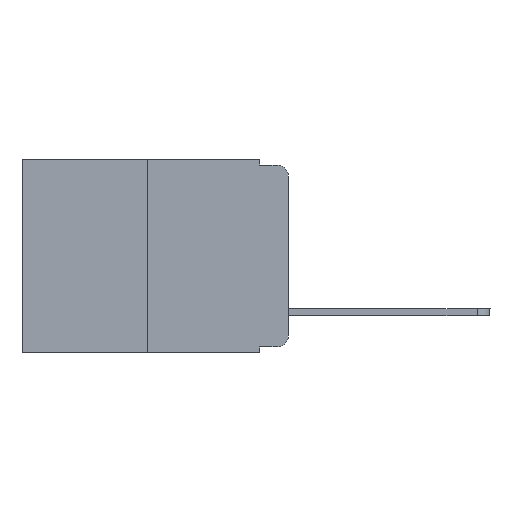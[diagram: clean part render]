
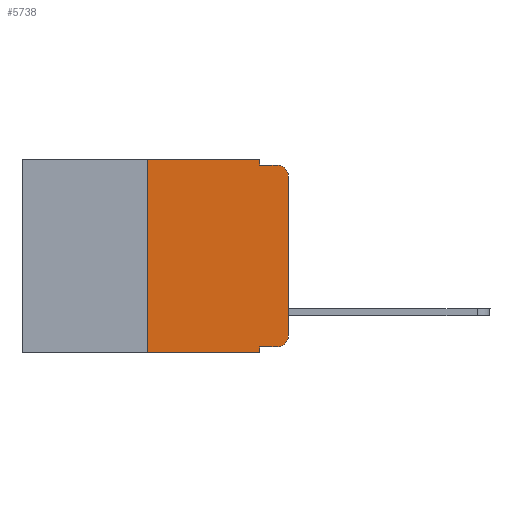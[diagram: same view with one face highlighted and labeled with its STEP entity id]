
A CAD part, left-side view. The second image highlights one B-rep face of the part: STEP entity #5738.
In plain terms, the highlighted planar face has unit normal (-1, 0, 0).
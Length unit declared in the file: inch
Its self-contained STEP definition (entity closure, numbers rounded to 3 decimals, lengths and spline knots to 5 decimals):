
#216 = EDGE_LOOP ( 'NONE', ( #12661, #5060, #540, #6950, #2958, #3601, #13389, #7223, #9988, #9364 ) ) ;
#259 = VECTOR ( 'NONE', #4154, 39.37008 ) ;
#318 = LINE ( 'NONE', #15858, #13446 ) ;
#540 = ORIENTED_EDGE ( 'NONE', *, *, #12259, .F. ) ;
#724 = VECTOR ( 'NONE', #11496, 39.37008 ) ;
#1175 = VERTEX_POINT ( 'NONE', #9957 ) ;
#1369 = VERTEX_POINT ( 'NONE', #2977 ) ;
#1578 = CARTESIAN_POINT ( 'NONE',  ( 0., 0.051, -0.01 ) ) ;
#1842 = EDGE_CURVE ( 'NONE', #11003, #3989, #5611, .T. ) ;
#2008 = LINE ( 'NONE', #15488, #11541 ) ;
#2069 = EDGE_CURVE ( 'NONE', #1369, #3989, #2008, .T. ) ;
#2119 = CARTESIAN_POINT ( 'NONE',  ( 0., 0.473, 0. ) ) ;
#2423 = DIRECTION ( 'NONE',  ( 0., -1., 0. ) ) ;
#2655 = AXIS2_PLACEMENT_3D ( 'NONE', #3126, #9514, #8325 ) ;
#2958 = ORIENTED_EDGE ( 'NONE', *, *, #6372, .F. ) ;
#2977 = CARTESIAN_POINT ( 'NONE',  ( 0., 0.25, -0.343 ) ) ;
#3126 = CARTESIAN_POINT ( 'NONE',  ( 0., 0.473, 0. ) ) ;
#3212 = DIRECTION ( 'NONE',  ( -1., 0., 0. ) ) ;
#3385 = DIRECTION ( 'NONE',  ( 0., 0., -1. ) ) ;
#3504 = DIRECTION ( 'NONE',  ( 0., 0., -1. ) ) ;
#3601 = ORIENTED_EDGE ( 'NONE', *, *, #12335, .F. ) ;
#3795 = VECTOR ( 'NONE', #4700, 39.37008 ) ;
#3989 = VERTEX_POINT ( 'NONE', #10804 ) ;
#4024 = CARTESIAN_POINT ( 'NONE',  ( 0., 0.051, -0.01 ) ) ;
#4154 = DIRECTION ( 'NONE',  ( 0., 0., -1. ) ) ;
#4359 = VECTOR ( 'NONE', #12160, 39.37008 ) ;
#4415 = CARTESIAN_POINT ( 'NONE',  ( 0., 0., -0.03 ) ) ;
#4562 = EDGE_CURVE ( 'NONE', #11003, #16370, #15292, .T. ) ;
#4700 = DIRECTION ( 'NONE',  ( 0., -1., 0. ) ) ;
#5060 = ORIENTED_EDGE ( 'NONE', *, *, #9894, .T. ) ;
#5487 = DIRECTION ( 'NONE',  ( -1., 0., 0. ) ) ;
#5527 = CARTESIAN_POINT ( 'NONE',  ( 0., 0.051, 0. ) ) ;
#5611 = LINE ( 'NONE', #5527, #259 ) ;
#5738 = ADVANCED_FACE ( 'NONE', ( #8158 ), #16005, .F. ) ;
#5801 = CARTESIAN_POINT ( 'NONE',  ( 0., 0., 0. ) ) ;
#6224 = CARTESIAN_POINT ( 'NONE',  ( 0., 0.25, 0. ) ) ;
#6372 = EDGE_CURVE ( 'NONE', #11596, #1175, #10990, .T. ) ;
#6851 = EDGE_CURVE ( 'NONE', #13293, #8648, #9861, .T. ) ;
#6950 = ORIENTED_EDGE ( 'NONE', *, *, #13025, .F. ) ;
#7210 = DIRECTION ( 'NONE',  ( 0., 0., 1. ) ) ;
#7223 = ORIENTED_EDGE ( 'NONE', *, *, #1842, .F. ) ;
#7736 = CARTESIAN_POINT ( 'NONE',  ( 0., 0., -0.313 ) ) ;
#8034 = CIRCLE ( 'NONE', #11540, 0.02 ) ;
#8158 = FACE_OUTER_BOUND ( 'NONE', #216, .T. ) ;
#8325 = DIRECTION ( 'NONE',  ( 0., 0., -1. ) ) ;
#8648 = VERTEX_POINT ( 'NONE', #4415 ) ;
#8885 = CARTESIAN_POINT ( 'NONE',  ( 0., 0.051, -0.333 ) ) ;
#9078 = VECTOR ( 'NONE', #16246, 39.37008 ) ;
#9087 = CARTESIAN_POINT ( 'NONE',  ( 0., 0.02, -0.01 ) ) ;
#9364 = ORIENTED_EDGE ( 'NONE', *, *, #15581, .T. ) ;
#9514 = DIRECTION ( 'NONE',  ( 1., 0., 0. ) ) ;
#9616 = DIRECTION ( 'NONE',  ( 0., 0., -1. ) ) ;
#9861 = LINE ( 'NONE', #5801, #4359 ) ;
#9894 = EDGE_CURVE ( 'NONE', #8648, #11940, #15010, .T. ) ;
#9957 = CARTESIAN_POINT ( 'NONE',  ( 0., 0.051, 0. ) ) ;
#9988 = ORIENTED_EDGE ( 'NONE', *, *, #4562, .T. ) ;
#10804 = CARTESIAN_POINT ( 'NONE',  ( 0., 0.051, -0.343 ) ) ;
#10867 = CARTESIAN_POINT ( 'NONE',  ( 0., 0.25, 0. ) ) ;
#10990 = LINE ( 'NONE', #2119, #3795 ) ;
#11003 = VERTEX_POINT ( 'NONE', #16224 ) ;
#11111 = CARTESIAN_POINT ( 'NONE',  ( 0., 0.02, -0.03 ) ) ;
#11496 = DIRECTION ( 'NONE',  ( 0., -1., 0. ) ) ;
#11540 = AXIS2_PLACEMENT_3D ( 'NONE', #14097, #5487, #3504 ) ;
#11541 = VECTOR ( 'NONE', #2423, 39.37008 ) ;
#11596 = VERTEX_POINT ( 'NONE', #6224 ) ;
#11940 = VERTEX_POINT ( 'NONE', #9087 ) ;
#12160 = DIRECTION ( 'NONE',  ( 0., 0., 1. ) ) ;
#12259 = EDGE_CURVE ( 'NONE', #14093, #11940, #13250, .T. ) ;
#12335 = EDGE_CURVE ( 'NONE', #1369, #11596, #15143, .T. ) ;
#12661 = ORIENTED_EDGE ( 'NONE', *, *, #6851, .T. ) ;
#13025 = EDGE_CURVE ( 'NONE', #1175, #14093, #318, .T. ) ;
#13250 = LINE ( 'NONE', #1578, #9078 ) ;
#13293 = VERTEX_POINT ( 'NONE', #7736 ) ;
#13389 = ORIENTED_EDGE ( 'NONE', *, *, #2069, .T. ) ;
#13446 = VECTOR ( 'NONE', #9616, 39.37008 ) ;
#13994 = VECTOR ( 'NONE', #7210, 39.37008 ) ;
#14093 = VERTEX_POINT ( 'NONE', #4024 ) ;
#14097 = CARTESIAN_POINT ( 'NONE',  ( 0., 0.02, -0.313 ) ) ;
#14447 = AXIS2_PLACEMENT_3D ( 'NONE', #11111, #3212, #3385 ) ;
#15010 = CIRCLE ( 'NONE', #14447, 0.02 ) ;
#15143 = LINE ( 'NONE', #10867, #13994 ) ;
#15292 = LINE ( 'NONE', #8885, #724 ) ;
#15346 = CARTESIAN_POINT ( 'NONE',  ( 0., 0.02, -0.333 ) ) ;
#15488 = CARTESIAN_POINT ( 'NONE',  ( 0., 0.473, -0.343 ) ) ;
#15581 = EDGE_CURVE ( 'NONE', #16370, #13293, #8034, .T. ) ;
#15858 = CARTESIAN_POINT ( 'NONE',  ( 0., 0.051, 0. ) ) ;
#16005 = PLANE ( 'NONE',  #2655 ) ;
#16224 = CARTESIAN_POINT ( 'NONE',  ( 0., 0.051, -0.333 ) ) ;
#16246 = DIRECTION ( 'NONE',  ( 0., -1., 0. ) ) ;
#16370 = VERTEX_POINT ( 'NONE', #15346 ) ;
